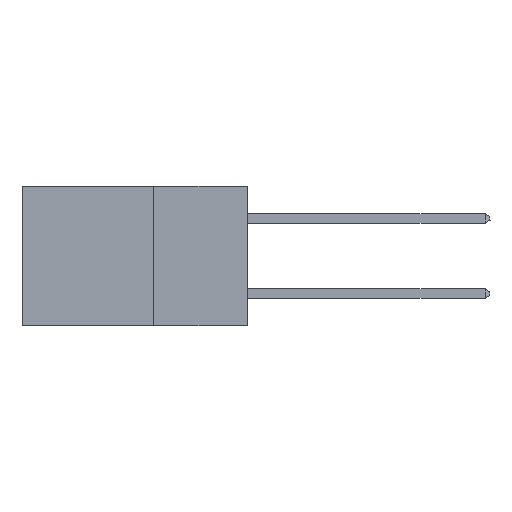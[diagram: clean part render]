
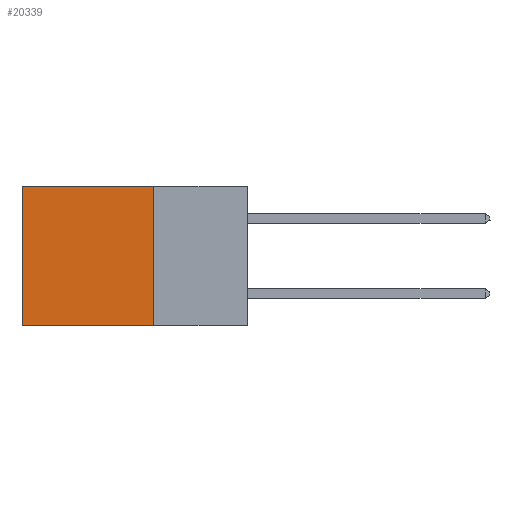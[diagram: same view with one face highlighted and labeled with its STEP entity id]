
A CAD part, left-side view. The second image highlights one B-rep face of the part: STEP entity #20339.
In plain terms, the highlighted planar face has unit normal (-1, 0, 0).
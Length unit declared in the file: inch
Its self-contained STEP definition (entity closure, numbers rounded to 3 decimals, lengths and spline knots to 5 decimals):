
#565 = EDGE_LOOP ( 'NONE', ( #31088, #22456, #18929, #14696 ) ) ;
#1523 = LINE ( 'NONE', #25115, #22050 ) ;
#3223 = DIRECTION ( 'NONE',  ( 0., 1., 0. ) ) ;
#5525 = VERTEX_POINT ( 'NONE', #14464 ) ;
#6698 = CARTESIAN_POINT ( 'NONE',  ( 0.298, 0.25, -0.37 ) ) ;
#8725 = CARTESIAN_POINT ( 'NONE',  ( 0.298, 0.25, 0. ) ) ;
#8794 = CARTESIAN_POINT ( 'NONE',  ( 0.298, 0.6, 0. ) ) ;
#9544 = VERTEX_POINT ( 'NONE', #6698 ) ;
#9822 = EDGE_CURVE ( 'NONE', #9544, #22909, #1523, .T. ) ;
#10038 = VECTOR ( 'NONE', #15009, 39.37008 ) ;
#10523 = EDGE_CURVE ( 'NONE', #5525, #9544, #23598, .T. ) ;
#11811 = CARTESIAN_POINT ( 'NONE',  ( 0.298, 0.25, 0. ) ) ;
#12816 = VECTOR ( 'NONE', #25535, 39.37008 ) ;
#13932 = VECTOR ( 'NONE', #24337, 39.37008 ) ;
#14464 = CARTESIAN_POINT ( 'NONE',  ( 0.298, 0.25, 0. ) ) ;
#14696 = ORIENTED_EDGE ( 'NONE', *, *, #22584, .T. ) ;
#15009 = DIRECTION ( 'NONE',  ( 0., 0., -1. ) ) ;
#15054 = LINE ( 'NONE', #24811, #10038 ) ;
#15516 = CARTESIAN_POINT ( 'NONE',  ( 0.298, 0.6, -0.37 ) ) ;
#17468 = LINE ( 'NONE', #8725, #12816 ) ;
#17599 = FACE_OUTER_BOUND ( 'NONE', #565, .T. ) ;
#18929 = ORIENTED_EDGE ( 'NONE', *, *, #10523, .F. ) ;
#19321 = PLANE ( 'NONE',  #25162 ) ;
#20339 = ADVANCED_FACE ( 'NONE', ( #17599 ), #19321, .F. ) ;
#21571 = DIRECTION ( 'NONE',  ( 1., 0., 0. ) ) ;
#22050 = VECTOR ( 'NONE', #3223, 39.37008 ) ;
#22456 = ORIENTED_EDGE ( 'NONE', *, *, #9822, .F. ) ;
#22584 = EDGE_CURVE ( 'NONE', #5525, #27340, #17468, .T. ) ;
#22909 = VERTEX_POINT ( 'NONE', #15516 ) ;
#23412 = EDGE_CURVE ( 'NONE', #27340, #22909, #15054, .T. ) ;
#23598 = LINE ( 'NONE', #11811, #13932 ) ;
#24337 = DIRECTION ( 'NONE',  ( 0., 0., -1. ) ) ;
#24811 = CARTESIAN_POINT ( 'NONE',  ( 0.298, 0.6, 0. ) ) ;
#25115 = CARTESIAN_POINT ( 'NONE',  ( 0.298, 0.25, -0.37 ) ) ;
#25162 = AXIS2_PLACEMENT_3D ( 'NONE', #26483, #21571, #31644 ) ;
#25535 = DIRECTION ( 'NONE',  ( 0., 1., 0. ) ) ;
#26483 = CARTESIAN_POINT ( 'NONE',  ( 0.298, 0.25, 0. ) ) ;
#27340 = VERTEX_POINT ( 'NONE', #8794 ) ;
#31088 = ORIENTED_EDGE ( 'NONE', *, *, #23412, .T. ) ;
#31644 = DIRECTION ( 'NONE',  ( 0., 0., -1. ) ) ;
